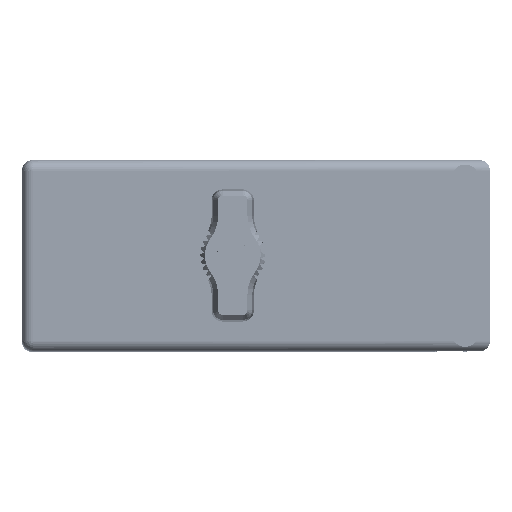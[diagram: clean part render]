
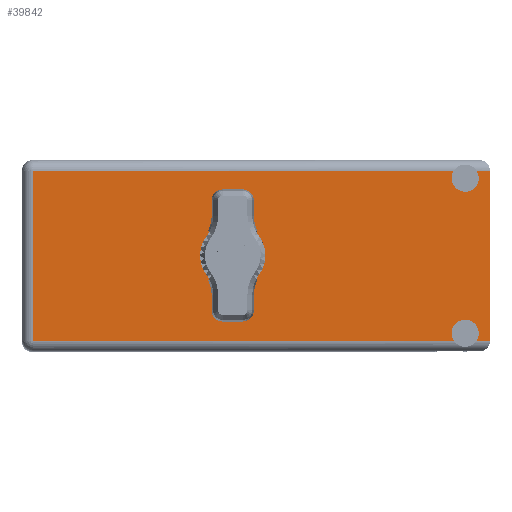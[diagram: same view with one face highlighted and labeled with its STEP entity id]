
A CAD part, top view. The second image highlights one B-rep face of the part: STEP entity #39842.
In plain terms, the highlighted face is planar.
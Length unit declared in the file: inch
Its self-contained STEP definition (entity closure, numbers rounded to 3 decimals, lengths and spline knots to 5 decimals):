
#358 = VERTEX_POINT ( 'NONE', #82861 ) ;
#1578 = AXIS2_PLACEMENT_3D ( 'NONE', #36437, #43470, #35459 ) ;
#2116 = LINE ( 'NONE', #51394, #95067 ) ;
#3062 = CARTESIAN_POINT ( 'NONE',  ( 0.07, 1.775, -1.164 ) ) ;
#3097 = LINE ( 'NONE', #75574, #68729 ) ;
#3419 = EDGE_CURVE ( 'NONE', #15646, #42616, #2116, .T. ) ;
#3743 = ORIENTED_EDGE ( 'NONE', *, *, #64039, .T. ) ;
#5159 = DIRECTION ( 'NONE',  ( 0., 0., 1. ) ) ;
#6544 = CARTESIAN_POINT ( 'NONE',  ( 0.07, 1.775, -0.07 ) ) ;
#7591 = EDGE_CURVE ( 'NONE', #55858, #22131, #31239, .T. ) ;
#8201 = CARTESIAN_POINT ( 'NONE',  ( 2.858, 1.775, -1.0295 ) ) ;
#11154 = ORIENTED_EDGE ( 'NONE', *, *, #47857, .F. ) ;
#14255 = CARTESIAN_POINT ( 'NONE',  ( 2.858, 1.775, -1.117 ) ) ;
#15646 = VERTEX_POINT ( 'NONE', #38030 ) ;
#16539 = VERTEX_POINT ( 'NONE', #38716 ) ;
#17389 = CIRCLE ( 'NONE', #57697, 0.0875 ) ;
#20422 = DIRECTION ( 'NONE',  ( 0., 1., 0. ) ) ;
#20947 = PLANE ( 'NONE',  #21430 ) ;
#21430 = AXIS2_PLACEMENT_3D ( 'NONE', #44608, #97974, #75277 ) ;
#22131 = VERTEX_POINT ( 'NONE', #85929 ) ;
#22468 = LINE ( 'NONE', #77518, #85683 ) ;
#23642 = AXIS2_PLACEMENT_3D ( 'NONE', #98248, #52604, #52927 ) ;
#24536 = EDGE_CURVE ( 'NONE', #33787, #358, #27020, .T. ) ;
#25346 = DIRECTION ( 'NONE',  ( -1., 0., 0. ) ) ;
#25447 = EDGE_CURVE ( 'NONE', #65131, #57890, #17389, .T. ) ;
#27020 = LINE ( 'NONE', #86659, #83108 ) ;
#27362 = ORIENTED_EDGE ( 'NONE', *, *, #54781, .F. ) ;
#27843 = ORIENTED_EDGE ( 'NONE', *, *, #25447, .F. ) ;
#30008 = VECTOR ( 'NONE', #60789, 39.37008 ) ;
#31239 = CIRCLE ( 'NONE', #42254, 0.125 ) ;
#31324 = EDGE_CURVE ( 'NONE', #97295, #42861, #22468, .T. ) ;
#33630 = EDGE_CURVE ( 'NONE', #22131, #55858, #78020, .T. ) ;
#33787 = VERTEX_POINT ( 'NONE', #85159 ) ;
#33817 = VERTEX_POINT ( 'NONE', #8201 ) ;
#34142 = ORIENTED_EDGE ( 'NONE', *, *, #33630, .F. ) ;
#35459 = DIRECTION ( 'NONE',  ( 0., 0., 1. ) ) ;
#36437 = CARTESIAN_POINT ( 'NONE',  ( 2.858, 1.775, -0.117 ) ) ;
#37700 = CARTESIAN_POINT ( 'NONE',  ( 0., 1.775, -1.164 ) ) ;
#38030 = CARTESIAN_POINT ( 'NONE',  ( 2.93181, 1.775, -0.07 ) ) ;
#38716 = CARTESIAN_POINT ( 'NONE',  ( 2.78419, 1.775, -1.164 ) ) ;
#39842 = ADVANCED_FACE ( 'NONE', ( #97307, #61587 ), #20947, .T. ) ;
#40723 = CARTESIAN_POINT ( 'NONE',  ( 2.858, 1.775, -1.117 ) ) ;
#41147 = EDGE_CURVE ( 'NONE', #16539, #97295, #46830, .T. ) ;
#42254 = AXIS2_PLACEMENT_3D ( 'NONE', #50498, #58873, #5159 ) ;
#42616 = VERTEX_POINT ( 'NONE', #71949 ) ;
#42861 = VERTEX_POINT ( 'NONE', #6544 ) ;
#43470 = DIRECTION ( 'NONE',  ( 0., 1., 0. ) ) ;
#43791 = ORIENTED_EDGE ( 'NONE', *, *, #41147, .T. ) ;
#44608 = CARTESIAN_POINT ( 'NONE',  ( 0., 1.775, -1.234 ) ) ;
#46830 = LINE ( 'NONE', #37700, #30008 ) ;
#47857 = EDGE_CURVE ( 'NONE', #33787, #42616, #83933, .T. ) ;
#49216 = ORIENTED_EDGE ( 'NONE', *, *, #24536, .T. ) ;
#50498 = CARTESIAN_POINT ( 'NONE',  ( 1.359, 1.775, -0.617 ) ) ;
#51394 = CARTESIAN_POINT ( 'NONE',  ( 3.018, 1.775, -0.07 ) ) ;
#52604 = DIRECTION ( 'NONE',  ( 0., 1., 0. ) ) ;
#52927 = DIRECTION ( 'NONE',  ( 0., 0., 1. ) ) ;
#53550 = CIRCLE ( 'NONE', #1578, 0.0875 ) ;
#53985 = ORIENTED_EDGE ( 'NONE', *, *, #86221, .F. ) ;
#54781 = EDGE_CURVE ( 'NONE', #15646, #65131, #53550, .T. ) ;
#55858 = VERTEX_POINT ( 'NONE', #71266 ) ;
#57113 = ORIENTED_EDGE ( 'NONE', *, *, #7591, .F. ) ;
#57697 = AXIS2_PLACEMENT_3D ( 'NONE', #66148, #20422, #73769 ) ;
#57890 = VERTEX_POINT ( 'NONE', #65041 ) ;
#58873 = DIRECTION ( 'NONE',  ( 0., 1., 0. ) ) ;
#59004 = AXIS2_PLACEMENT_3D ( 'NONE', #14255, #90893, #68923 ) ;
#60789 = DIRECTION ( 'NONE',  ( -1., 0., 0. ) ) ;
#61587 = FACE_OUTER_BOUND ( 'NONE', #63652, .T. ) ;
#62080 = AXIS2_PLACEMENT_3D ( 'NONE', #40723, #78687, #93064 ) ;
#62205 = ORIENTED_EDGE ( 'NONE', *, *, #3419, .T. ) ;
#63076 = CIRCLE ( 'NONE', #62080, 0.0875 ) ;
#63135 = ORIENTED_EDGE ( 'NONE', *, *, #31324, .T. ) ;
#63652 = EDGE_LOOP ( 'NONE', ( #3743, #27843, #27362, #62205, #11154, #49216, #53985, #86159, #43791, #63135 ) ) ;
#63733 = VECTOR ( 'NONE', #92895, 39.37008 ) ;
#64039 = EDGE_CURVE ( 'NONE', #42861, #57890, #3097, .T. ) ;
#65041 = CARTESIAN_POINT ( 'NONE',  ( 2.78419, 1.775, -0.07 ) ) ;
#65131 = VERTEX_POINT ( 'NONE', #84199 ) ;
#66148 = CARTESIAN_POINT ( 'NONE',  ( 2.858, 1.775, -0.117 ) ) ;
#68729 = VECTOR ( 'NONE', #83211, 39.37008 ) ;
#68923 = DIRECTION ( 'NONE',  ( 0., 0., 1. ) ) ;
#69857 = DIRECTION ( 'NONE',  ( 0., 0., 1. ) ) ;
#70965 = EDGE_CURVE ( 'NONE', #16539, #33817, #63076, .T. ) ;
#71266 = CARTESIAN_POINT ( 'NONE',  ( 1.359, 1.775, -0.492 ) ) ;
#71949 = CARTESIAN_POINT ( 'NONE',  ( 3.018, 1.775, -0.07 ) ) ;
#73769 = DIRECTION ( 'NONE',  ( 0., 0., 1. ) ) ;
#75277 = DIRECTION ( 'NONE',  ( 0., 0., 1. ) ) ;
#75574 = CARTESIAN_POINT ( 'NONE',  ( 3.018, 1.775, -0.07 ) ) ;
#77234 = CARTESIAN_POINT ( 'NONE',  ( 3.018, 1.775, 0. ) ) ;
#77518 = CARTESIAN_POINT ( 'NONE',  ( 0.07, 1.775, -1.234 ) ) ;
#78020 = CIRCLE ( 'NONE', #23642, 0.125 ) ;
#78687 = DIRECTION ( 'NONE',  ( 0., 1., 0. ) ) ;
#82005 = DIRECTION ( 'NONE',  ( 1., 0., 0. ) ) ;
#82861 = CARTESIAN_POINT ( 'NONE',  ( 2.93181, 1.775, -1.164 ) ) ;
#83108 = VECTOR ( 'NONE', #25346, 39.37008 ) ;
#83211 = DIRECTION ( 'NONE',  ( 1., 0., 0. ) ) ;
#83933 = LINE ( 'NONE', #77234, #63733 ) ;
#84199 = CARTESIAN_POINT ( 'NONE',  ( 2.858, 1.775, -0.2045 ) ) ;
#85159 = CARTESIAN_POINT ( 'NONE',  ( 3.018, 1.775, -1.164 ) ) ;
#85683 = VECTOR ( 'NONE', #69857, 39.37008 ) ;
#85929 = CARTESIAN_POINT ( 'NONE',  ( 1.359, 1.775, -0.742 ) ) ;
#86159 = ORIENTED_EDGE ( 'NONE', *, *, #70965, .F. ) ;
#86221 = EDGE_CURVE ( 'NONE', #33817, #358, #87134, .T. ) ;
#86659 = CARTESIAN_POINT ( 'NONE',  ( 0., 1.775, -1.164 ) ) ;
#87134 = CIRCLE ( 'NONE', #59004, 0.0875 ) ;
#90893 = DIRECTION ( 'NONE',  ( 0., 1., 0. ) ) ;
#91704 = EDGE_LOOP ( 'NONE', ( #57113, #34142 ) ) ;
#92895 = DIRECTION ( 'NONE',  ( 0., 0., 1. ) ) ;
#93064 = DIRECTION ( 'NONE',  ( 0., 0., 1. ) ) ;
#95067 = VECTOR ( 'NONE', #82005, 39.37008 ) ;
#97295 = VERTEX_POINT ( 'NONE', #3062 ) ;
#97307 = FACE_BOUND ( 'NONE', #91704, .T. ) ;
#97974 = DIRECTION ( 'NONE',  ( 0., 1., 0. ) ) ;
#98248 = CARTESIAN_POINT ( 'NONE',  ( 1.359, 1.775, -0.617 ) ) ;
